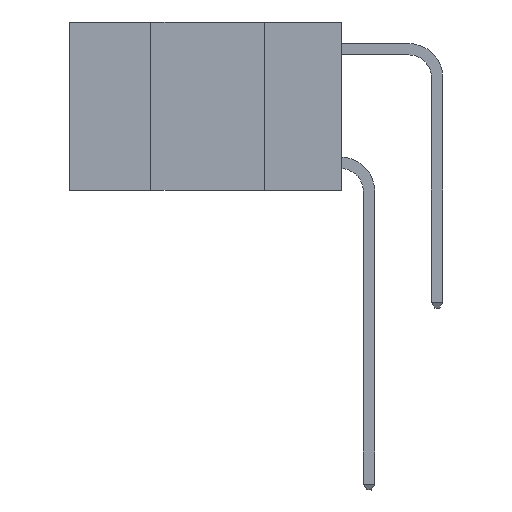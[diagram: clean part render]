
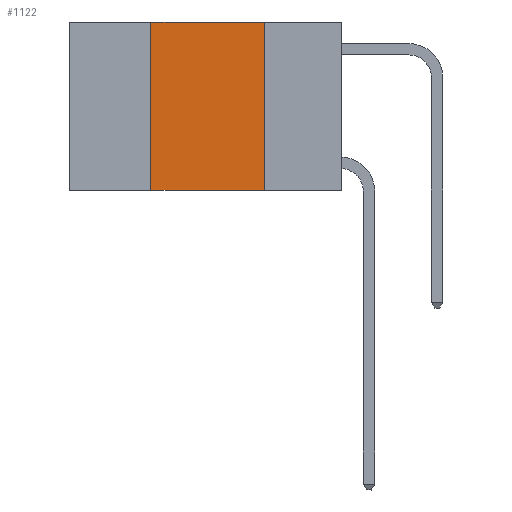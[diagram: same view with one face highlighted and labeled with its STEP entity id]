
A CAD part, left-side view. The second image highlights one B-rep face of the part: STEP entity #1122.
In plain terms, the highlighted planar face has unit normal (-1, 0, 0).
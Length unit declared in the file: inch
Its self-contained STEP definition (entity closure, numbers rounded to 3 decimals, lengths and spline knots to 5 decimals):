
#324 = DIRECTION ( 'NONE',  ( 0., -1., 0. ) ) ;
#656 = PLANE ( 'NONE',  #17974 ) ;
#669 = CARTESIAN_POINT ( 'NONE',  ( 0., 0.17, 0. ) ) ;
#743 = DIRECTION ( 'NONE',  ( 0., 0., 1. ) ) ;
#1122 = ADVANCED_FACE ( 'NONE', ( #24173 ), #656, .F. ) ;
#1180 = EDGE_CURVE ( 'NONE', #10996, #24829, #8090, .T. ) ;
#2446 = CARTESIAN_POINT ( 'NONE',  ( 0., 0.6, 0. ) ) ;
#2644 = DIRECTION ( 'NONE',  ( 0., 0., -1. ) ) ;
#6279 = CARTESIAN_POINT ( 'NONE',  ( 0., 0.42, 0. ) ) ;
#7479 = VECTOR ( 'NONE', #743, 39.37008 ) ;
#8090 = LINE ( 'NONE', #23671, #7479 ) ;
#9602 = LINE ( 'NONE', #11781, #24460 ) ;
#10996 = VERTEX_POINT ( 'NONE', #23280 ) ;
#11781 = CARTESIAN_POINT ( 'NONE',  ( 0., 0.17, 0. ) ) ;
#12355 = CARTESIAN_POINT ( 'NONE',  ( 0., 0.6, 0. ) ) ;
#13401 = LINE ( 'NONE', #2446, #17986 ) ;
#13735 = DIRECTION ( 'NONE',  ( 0., 0., -1. ) ) ;
#14327 = DIRECTION ( 'NONE',  ( 1., 0., 0. ) ) ;
#15992 = EDGE_LOOP ( 'NONE', ( #16316, #21467, #21228, #19218 ) ) ;
#16316 = ORIENTED_EDGE ( 'NONE', *, *, #18955, .F. ) ;
#17974 = AXIS2_PLACEMENT_3D ( 'NONE', #12355, #14327, #2644 ) ;
#17986 = VECTOR ( 'NONE', #18039, 39.37008 ) ;
#18039 = DIRECTION ( 'NONE',  ( 0., -1., 0. ) ) ;
#18859 = VECTOR ( 'NONE', #324, 39.37008 ) ;
#18955 = EDGE_CURVE ( 'NONE', #24953, #21751, #9602, .T. ) ;
#19218 = ORIENTED_EDGE ( 'NONE', *, *, #20632, .T. ) ;
#19804 = CARTESIAN_POINT ( 'NONE',  ( 0., 0.6, -0.37 ) ) ;
#19975 = EDGE_CURVE ( 'NONE', #24829, #24953, #13401, .T. ) ;
#20632 = EDGE_CURVE ( 'NONE', #10996, #21751, #24001, .T. ) ;
#21228 = ORIENTED_EDGE ( 'NONE', *, *, #1180, .F. ) ;
#21467 = ORIENTED_EDGE ( 'NONE', *, *, #19975, .F. ) ;
#21751 = VERTEX_POINT ( 'NONE', #23195 ) ;
#23195 = CARTESIAN_POINT ( 'NONE',  ( 0., 0.17, -0.37 ) ) ;
#23280 = CARTESIAN_POINT ( 'NONE',  ( 0., 0.42, -0.37 ) ) ;
#23671 = CARTESIAN_POINT ( 'NONE',  ( 0., 0.42, 0. ) ) ;
#24001 = LINE ( 'NONE', #19804, #18859 ) ;
#24173 = FACE_OUTER_BOUND ( 'NONE', #15992, .T. ) ;
#24460 = VECTOR ( 'NONE', #13735, 39.37008 ) ;
#24829 = VERTEX_POINT ( 'NONE', #6279 ) ;
#24953 = VERTEX_POINT ( 'NONE', #669 ) ;
